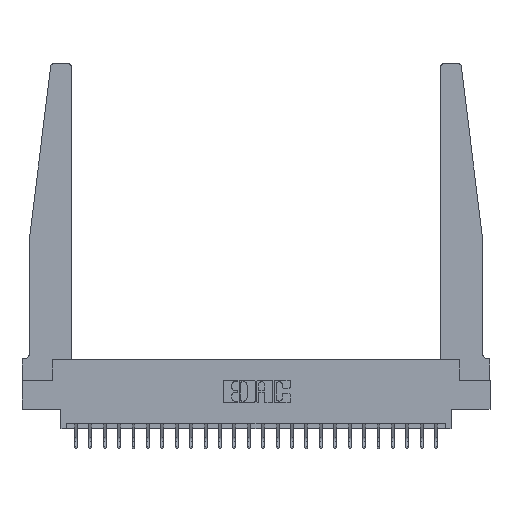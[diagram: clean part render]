
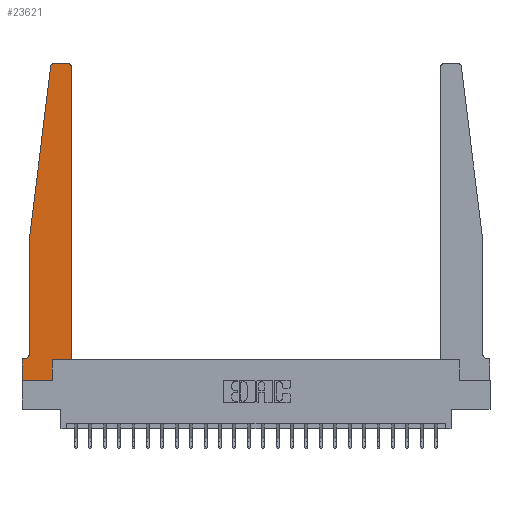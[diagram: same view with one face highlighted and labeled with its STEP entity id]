
A CAD part, top view. The second image highlights one B-rep face of the part: STEP entity #23621.
In plain terms, the highlighted planar face has unit normal (0, 0, 1).
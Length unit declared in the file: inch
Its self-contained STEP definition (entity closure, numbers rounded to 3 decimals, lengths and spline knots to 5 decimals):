
#233 = LINE ( 'NONE', #23113, #11473 ) ;
#363 = DIRECTION ( 'NONE',  ( -1., 0., 0. ) ) ;
#366 = AXIS2_PLACEMENT_3D ( 'NONE', #13391, #17381, #13765 ) ;
#516 = CARTESIAN_POINT ( 'NONE',  ( 0., 0., 0.37 ) ) ;
#726 = CARTESIAN_POINT ( 'NONE',  ( 0.425, 0.18, 0.37 ) ) ;
#855 = CARTESIAN_POINT ( 'NONE',  ( 0.2605, 0.18, 0.37 ) ) ;
#2157 = LINE ( 'NONE', #22784, #23071 ) ;
#2365 = FACE_OUTER_BOUND ( 'NONE', #15745, .T. ) ;
#2661 = ORIENTED_EDGE ( 'NONE', *, *, #21167, .T. ) ;
#3045 = CARTESIAN_POINT ( 'NONE',  ( 0., 0.1875, 0.37 ) ) ;
#3333 = EDGE_CURVE ( 'NONE', #18153, #18968, #4718, .T. ) ;
#3934 = CARTESIAN_POINT ( 'NONE',  ( 0.015, 0.1875, 0.37 ) ) ;
#4127 = AXIS2_PLACEMENT_3D ( 'NONE', #23372, #23245, #363 ) ;
#4291 = CIRCLE ( 'NONE', #8285, 0.03 ) ;
#4718 = LINE ( 'NONE', #855, #21545 ) ;
#4903 = LINE ( 'NONE', #20277, #20121 ) ;
#5325 = CIRCLE ( 'NONE', #4127, 0.05 ) ;
#5393 = VERTEX_POINT ( 'NONE', #11456 ) ;
#5732 = ORIENTED_EDGE ( 'NONE', *, *, #17806, .T. ) ;
#5759 = CARTESIAN_POINT ( 'NONE',  ( 0.395, 2.72, 0.37 ) ) ;
#6006 = VERTEX_POINT ( 'NONE', #3934 ) ;
#6241 = DIRECTION ( 'NONE',  ( 0., 1., 0. ) ) ;
#6242 = LINE ( 'NONE', #18116, #9517 ) ;
#7083 = ORIENTED_EDGE ( 'NONE', *, *, #8457, .T. ) ;
#7758 = PLANE ( 'NONE',  #366 ) ;
#8168 = ORIENTED_EDGE ( 'NONE', *, *, #21266, .T. ) ;
#8285 = AXIS2_PLACEMENT_3D ( 'NONE', #20300, #14449, #11195 ) ;
#8340 = CARTESIAN_POINT ( 'NONE',  ( 0.2605, 0., 0.37 ) ) ;
#8414 = EDGE_CURVE ( 'NONE', #24657, #23791, #18683, .T. ) ;
#8457 = EDGE_CURVE ( 'NONE', #16777, #24657, #6242, .T. ) ;
#8465 = ORIENTED_EDGE ( 'NONE', *, *, #8414, .T. ) ;
#8896 = VERTEX_POINT ( 'NONE', #21705 ) ;
#9392 = VECTOR ( 'NONE', #20573, 39.37008 ) ;
#9517 = VECTOR ( 'NONE', #14126, 39.37008 ) ;
#10013 = DIRECTION ( 'NONE',  ( 0., 0., 1. ) ) ;
#10747 = EDGE_CURVE ( 'NONE', #13075, #19360, #17036, .T. ) ;
#10808 = ORIENTED_EDGE ( 'NONE', *, *, #14033, .T. ) ;
#10970 = LINE ( 'NONE', #16327, #9392 ) ;
#11195 = DIRECTION ( 'NONE',  ( 1., 0., 0. ) ) ;
#11456 = CARTESIAN_POINT ( 'NONE',  ( 0.24675, 2.72367, 0.37 ) ) ;
#11473 = VECTOR ( 'NONE', #20054, 39.37008 ) ;
#13075 = VERTEX_POINT ( 'NONE', #3045 ) ;
#13386 = LINE ( 'NONE', #17257, #20401 ) ;
#13391 = CARTESIAN_POINT ( 'NONE',  ( 0., 0.1875, 0.37 ) ) ;
#13401 = DIRECTION ( 'NONE',  ( 1., 0., 0. ) ) ;
#13765 = DIRECTION ( 'NONE',  ( 1., 0., 0. ) ) ;
#14033 = EDGE_CURVE ( 'NONE', #23791, #8896, #13386, .T. ) ;
#14126 = DIRECTION ( 'NONE',  ( 0., 1., 0. ) ) ;
#14449 = DIRECTION ( 'NONE',  ( 0., 0., 1. ) ) ;
#14920 = ORIENTED_EDGE ( 'NONE', *, *, #15166, .T. ) ;
#15166 = EDGE_CURVE ( 'NONE', #19360, #18153, #17645, .T. ) ;
#15249 = CARTESIAN_POINT ( 'NONE',  ( 0., 0., 0.37 ) ) ;
#15429 = CARTESIAN_POINT ( 'NONE',  ( 0.2605, 0.18, 0.37 ) ) ;
#15745 = EDGE_LOOP ( 'NONE', ( #10808, #8168, #20663, #18410, #21864, #2661, #22481, #14920, #21724, #5732, #7083, #8465 ) ) ;
#16327 = CARTESIAN_POINT ( 'NONE',  ( 0.065, 1.25, 0.37 ) ) ;
#16775 = EDGE_CURVE ( 'NONE', #17688, #6006, #5325, .T. ) ;
#16777 = VERTEX_POINT ( 'NONE', #726 ) ;
#17036 = LINE ( 'NONE', #17153, #17563 ) ;
#17153 = CARTESIAN_POINT ( 'NONE',  ( 0., 0., 0.37 ) ) ;
#17257 = CARTESIAN_POINT ( 'NONE',  ( 0.25, 2.75, 0.37 ) ) ;
#17381 = DIRECTION ( 'NONE',  ( 0., 0., 1. ) ) ;
#17563 = VECTOR ( 'NONE', #20757, 39.37008 ) ;
#17645 = LINE ( 'NONE', #516, #21220 ) ;
#17688 = VERTEX_POINT ( 'NONE', #17803 ) ;
#17803 = CARTESIAN_POINT ( 'NONE',  ( 0.065, 0.2375, 0.37 ) ) ;
#17806 = EDGE_CURVE ( 'NONE', #18968, #16777, #4903, .T. ) ;
#18116 = CARTESIAN_POINT ( 'NONE',  ( 0.425, 0.18, 0.37 ) ) ;
#18153 = VERTEX_POINT ( 'NONE', #8340 ) ;
#18281 = EDGE_CURVE ( 'NONE', #5393, #20179, #10970, .T. ) ;
#18410 = ORIENTED_EDGE ( 'NONE', *, *, #22058, .T. ) ;
#18484 = CARTESIAN_POINT ( 'NONE',  ( 0.395, 2.75, 0.37 ) ) ;
#18683 = CIRCLE ( 'NONE', #23862, 0.03 ) ;
#18968 = VERTEX_POINT ( 'NONE', #15429 ) ;
#19360 = VERTEX_POINT ( 'NONE', #15249 ) ;
#19605 = DIRECTION ( 'NONE',  ( -1., 0., 0. ) ) ;
#19639 = DIRECTION ( 'NONE',  ( 1., 0., 0. ) ) ;
#19794 = DIRECTION ( 'NONE',  ( 1., 0., 0. ) ) ;
#20054 = DIRECTION ( 'NONE',  ( -1., 0., 0. ) ) ;
#20121 = VECTOR ( 'NONE', #19794, 39.37008 ) ;
#20179 = VERTEX_POINT ( 'NONE', #20798 ) ;
#20277 = CARTESIAN_POINT ( 'NONE',  ( 0.425, 0.18, 0.37 ) ) ;
#20300 = CARTESIAN_POINT ( 'NONE',  ( 0.27653, 2.72, 0.37 ) ) ;
#20401 = VECTOR ( 'NONE', #19605, 39.37008 ) ;
#20573 = DIRECTION ( 'NONE',  ( -0.122, -0.992, 0. ) ) ;
#20663 = ORIENTED_EDGE ( 'NONE', *, *, #18281, .T. ) ;
#20757 = DIRECTION ( 'NONE',  ( 0., -1., 0. ) ) ;
#20798 = CARTESIAN_POINT ( 'NONE',  ( 0.065, 1.25, 0.37 ) ) ;
#21008 = DIRECTION ( 'NONE',  ( 0., -1., 0. ) ) ;
#21167 = EDGE_CURVE ( 'NONE', #6006, #13075, #233, .T. ) ;
#21220 = VECTOR ( 'NONE', #19639, 39.37008 ) ;
#21266 = EDGE_CURVE ( 'NONE', #8896, #5393, #4291, .T. ) ;
#21545 = VECTOR ( 'NONE', #6241, 39.37008 ) ;
#21705 = CARTESIAN_POINT ( 'NONE',  ( 0.27653, 2.75, 0.37 ) ) ;
#21724 = ORIENTED_EDGE ( 'NONE', *, *, #3333, .T. ) ;
#21864 = ORIENTED_EDGE ( 'NONE', *, *, #16775, .T. ) ;
#22058 = EDGE_CURVE ( 'NONE', #20179, #17688, #2157, .T. ) ;
#22375 = CARTESIAN_POINT ( 'NONE',  ( 0.425, 2.72, 0.37 ) ) ;
#22481 = ORIENTED_EDGE ( 'NONE', *, *, #10747, .T. ) ;
#22784 = CARTESIAN_POINT ( 'NONE',  ( 0.065, 1.25, 0.37 ) ) ;
#23071 = VECTOR ( 'NONE', #21008, 39.37008 ) ;
#23113 = CARTESIAN_POINT ( 'NONE',  ( 0.065, 0.1875, 0.37 ) ) ;
#23245 = DIRECTION ( 'NONE',  ( 0., 0., -1. ) ) ;
#23372 = CARTESIAN_POINT ( 'NONE',  ( 0.015, 0.2375, 0.37 ) ) ;
#23621 = ADVANCED_FACE ( 'NONE', ( #2365 ), #7758, .T. ) ;
#23791 = VERTEX_POINT ( 'NONE', #18484 ) ;
#23862 = AXIS2_PLACEMENT_3D ( 'NONE', #5759, #10013, #13401 ) ;
#24657 = VERTEX_POINT ( 'NONE', #22375 ) ;
